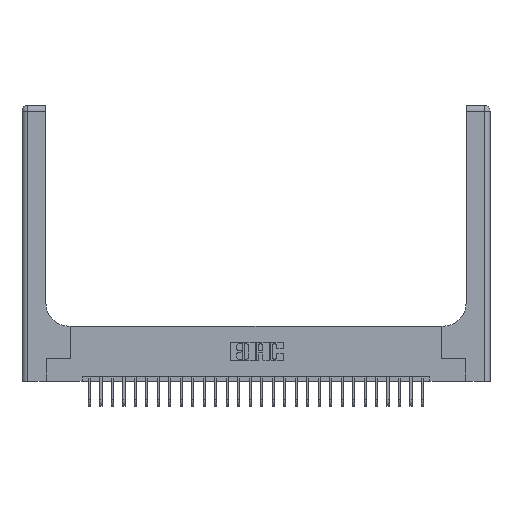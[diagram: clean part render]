
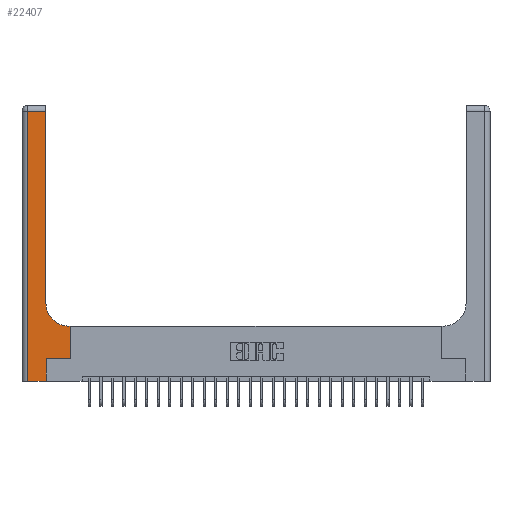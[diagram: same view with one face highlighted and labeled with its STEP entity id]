
A CAD part, top view. The second image highlights one B-rep face of the part: STEP entity #22407.
In plain terms, the highlighted planar face has unit normal (0, 0, 1).
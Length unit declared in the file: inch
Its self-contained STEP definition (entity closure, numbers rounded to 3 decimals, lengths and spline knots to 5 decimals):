
#207 = ORIENTED_EDGE ( 'NONE', *, *, #16366, .T. ) ;
#272 = VERTEX_POINT ( 'NONE', #20217 ) ;
#524 = VECTOR ( 'NONE', #18909, 39.37008 ) ;
#701 = LINE ( 'NONE', #2789, #4345 ) ;
#1124 = ORIENTED_EDGE ( 'NONE', *, *, #5558, .T. ) ;
#1286 = ORIENTED_EDGE ( 'NONE', *, *, #25305, .T. ) ;
#1539 = CARTESIAN_POINT ( 'NONE',  ( 0., 3., 0.37 ) ) ;
#1694 = EDGE_CURVE ( 'NONE', #2119, #272, #6947, .T. ) ;
#2119 = VERTEX_POINT ( 'NONE', #20811 ) ;
#2214 = VECTOR ( 'NONE', #8334, 39.37008 ) ;
#2339 = LINE ( 'NONE', #24875, #25667 ) ;
#2347 = CARTESIAN_POINT ( 'NONE',  ( 0., 0., 0.37 ) ) ;
#2493 = VERTEX_POINT ( 'NONE', #19900 ) ;
#2789 = CARTESIAN_POINT ( 'NONE',  ( 0., 2.94, 0.37 ) ) ;
#2903 = LINE ( 'NONE', #20994, #524 ) ;
#2909 = EDGE_LOOP ( 'NONE', ( #16141, #6682, #1286, #6568, #207, #3904, #25238, #1124, #16157 ) ) ;
#2977 = AXIS2_PLACEMENT_3D ( 'NONE', #1539, #9652, #5840 ) ;
#3048 = DIRECTION ( 'NONE',  ( -1., 0., 0. ) ) ;
#3222 = DIRECTION ( 'NONE',  ( 0., -1., 0. ) ) ;
#3273 = VERTEX_POINT ( 'NONE', #14410 ) ;
#3352 = DIRECTION ( 'NONE',  ( -1., 0., 0. ) ) ;
#3904 = ORIENTED_EDGE ( 'NONE', *, *, #25173, .T. ) ;
#4345 = VECTOR ( 'NONE', #3048, 39.37008 ) ;
#4641 = DIRECTION ( 'NONE',  ( 0., 0., -1. ) ) ;
#5252 = EDGE_CURVE ( 'NONE', #17508, #10444, #6243, .T. ) ;
#5435 = CARTESIAN_POINT ( 'NONE',  ( 0.26, 0.6, 0.37 ) ) ;
#5558 = EDGE_CURVE ( 'NONE', #20615, #6321, #23688, .T. ) ;
#5765 = EDGE_CURVE ( 'NONE', #6321, #2119, #10825, .T. ) ;
#5840 = DIRECTION ( 'NONE',  ( -1., 0., 0. ) ) ;
#6215 = AXIS2_PLACEMENT_3D ( 'NONE', #22998, #4641, #12640 ) ;
#6243 = LINE ( 'NONE', #2347, #16672 ) ;
#6321 = VERTEX_POINT ( 'NONE', #7865 ) ;
#6568 = ORIENTED_EDGE ( 'NONE', *, *, #5252, .T. ) ;
#6682 = ORIENTED_EDGE ( 'NONE', *, *, #18580, .T. ) ;
#6947 = LINE ( 'NONE', #18636, #12592 ) ;
#7425 = DIRECTION ( 'NONE',  ( 0., 1., 0. ) ) ;
#7865 = CARTESIAN_POINT ( 'NONE',  ( 0.51, 0.6, 0.37 ) ) ;
#8334 = DIRECTION ( 'NONE',  ( 1., 0., 0. ) ) ;
#8537 = DIRECTION ( 'NONE',  ( 0., 1., 0. ) ) ;
#8717 = CARTESIAN_POINT ( 'NONE',  ( 0.265, 0., 0.37 ) ) ;
#9168 = VERTEX_POINT ( 'NONE', #24722 ) ;
#9652 = DIRECTION ( 'NONE',  ( 0., 0., -1. ) ) ;
#10049 = DIRECTION ( 'NONE',  ( 1., 0., 0. ) ) ;
#10444 = VERTEX_POINT ( 'NONE', #8717 ) ;
#10825 = CIRCLE ( 'NONE', #6215, 0.25 ) ;
#11817 = CARTESIAN_POINT ( 'NONE',  ( 0.06, 0., 0.37 ) ) ;
#12066 = VECTOR ( 'NONE', #3352, 39.37008 ) ;
#12208 = VECTOR ( 'NONE', #7425, 39.37008 ) ;
#12592 = VECTOR ( 'NONE', #8537, 39.37008 ) ;
#12640 = DIRECTION ( 'NONE',  ( 1., 0., 0. ) ) ;
#14410 = CARTESIAN_POINT ( 'NONE',  ( 0.06, 2.94, 0.37 ) ) ;
#14682 = CARTESIAN_POINT ( 'NONE',  ( 0.528, 0.6, 0.37 ) ) ;
#16141 = ORIENTED_EDGE ( 'NONE', *, *, #1694, .T. ) ;
#16157 = ORIENTED_EDGE ( 'NONE', *, *, #5765, .T. ) ;
#16366 = EDGE_CURVE ( 'NONE', #10444, #2493, #23694, .T. ) ;
#16672 = VECTOR ( 'NONE', #10049, 39.37008 ) ;
#17096 = EDGE_CURVE ( 'NONE', #9168, #20615, #2903, .T. ) ;
#17419 = FACE_OUTER_BOUND ( 'NONE', #2909, .T. ) ;
#17508 = VERTEX_POINT ( 'NONE', #11817 ) ;
#17657 = CARTESIAN_POINT ( 'NONE',  ( 0.265, 0., 0.37 ) ) ;
#18324 = LINE ( 'NONE', #20541, #2214 ) ;
#18580 = EDGE_CURVE ( 'NONE', #272, #3273, #701, .T. ) ;
#18636 = CARTESIAN_POINT ( 'NONE',  ( 0.26, 3., 0.37 ) ) ;
#18909 = DIRECTION ( 'NONE',  ( 0., 1., 0. ) ) ;
#19900 = CARTESIAN_POINT ( 'NONE',  ( 0.265, 0.25, 0.37 ) ) ;
#20217 = CARTESIAN_POINT ( 'NONE',  ( 0.26, 2.94, 0.37 ) ) ;
#20541 = CARTESIAN_POINT ( 'NONE',  ( 0.265, 0.25, 0.37 ) ) ;
#20615 = VERTEX_POINT ( 'NONE', #14682 ) ;
#20811 = CARTESIAN_POINT ( 'NONE',  ( 0.26, 0.85, 0.37 ) ) ;
#20994 = CARTESIAN_POINT ( 'NONE',  ( 0.528, 0.25, 0.37 ) ) ;
#21611 = PLANE ( 'NONE',  #2977 ) ;
#22407 = ADVANCED_FACE ( 'NONE', ( #17419 ), #21611, .F. ) ;
#22998 = CARTESIAN_POINT ( 'NONE',  ( 0.51, 0.85, 0.37 ) ) ;
#23688 = LINE ( 'NONE', #5435, #12066 ) ;
#23694 = LINE ( 'NONE', #17657, #12208 ) ;
#24722 = CARTESIAN_POINT ( 'NONE',  ( 0.528, 0.25, 0.37 ) ) ;
#24875 = CARTESIAN_POINT ( 'NONE',  ( 0.06, 3., 0.37 ) ) ;
#25173 = EDGE_CURVE ( 'NONE', #2493, #9168, #18324, .T. ) ;
#25238 = ORIENTED_EDGE ( 'NONE', *, *, #17096, .T. ) ;
#25305 = EDGE_CURVE ( 'NONE', #3273, #17508, #2339, .T. ) ;
#25667 = VECTOR ( 'NONE', #3222, 39.37008 ) ;
